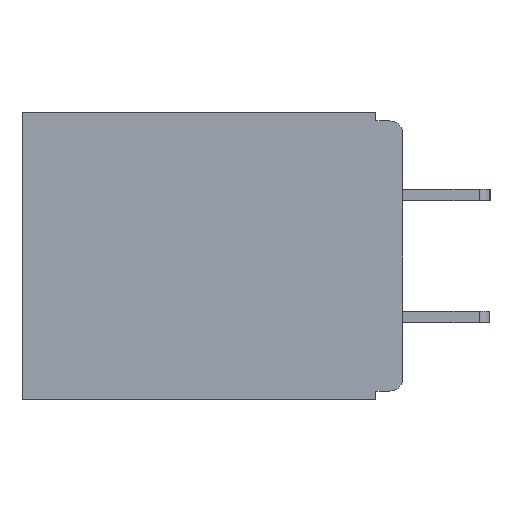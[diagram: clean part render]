
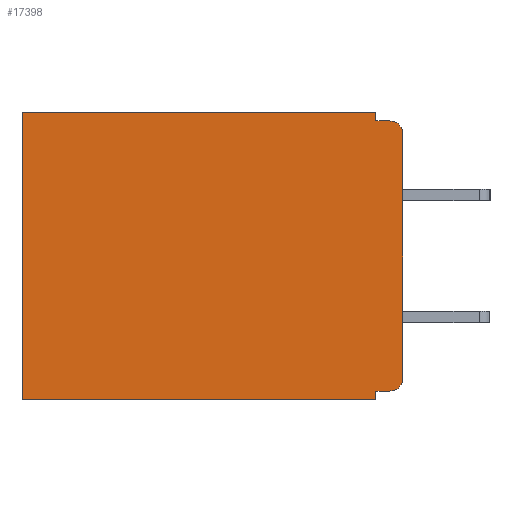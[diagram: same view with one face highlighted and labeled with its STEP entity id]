
A CAD part, left-side view. The second image highlights one B-rep face of the part: STEP entity #17398.
In plain terms, the highlighted planar face has unit normal (-1, 0, 0).
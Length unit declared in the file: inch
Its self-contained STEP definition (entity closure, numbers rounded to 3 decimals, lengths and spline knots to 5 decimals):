
#176 = CIRCLE ( 'NONE', #2695, 0.015 ) ;
#300 = ORIENTED_EDGE ( 'NONE', *, *, #22108, .F. ) ;
#583 = DIRECTION ( 'NONE',  ( 0., 0., -1. ) ) ;
#605 = DIRECTION ( 'NONE',  ( -1., 0., 0. ) ) ;
#666 = CARTESIAN_POINT ( 'NONE',  ( 0.3, 0.015, -0.305 ) ) ;
#902 = EDGE_CURVE ( 'NONE', #16992, #15504, #8045, .T. ) ;
#1127 = EDGE_CURVE ( 'NONE', #23476, #9948, #3181, .T. ) ;
#1251 = ORIENTED_EDGE ( 'NONE', *, *, #19569, .T. ) ;
#1346 = VECTOR ( 'NONE', #21164, 39.37008 ) ;
#1604 = CARTESIAN_POINT ( 'NONE',  ( 0.3, 0.015, -0.025 ) ) ;
#1906 = LINE ( 'NONE', #24030, #11576 ) ;
#1983 = VERTEX_POINT ( 'NONE', #21774 ) ;
#2018 = CARTESIAN_POINT ( 'NONE',  ( 0.3, 0., -0.32 ) ) ;
#2267 = VECTOR ( 'NONE', #6379, 39.37008 ) ;
#2303 = EDGE_LOOP ( 'NONE', ( #6532, #10044, #18871, #16533, #1251, #11111, #6105, #300, #2674, #8237 ) ) ;
#2674 = ORIENTED_EDGE ( 'NONE', *, *, #21019, .F. ) ;
#2695 = AXIS2_PLACEMENT_3D ( 'NONE', #666, #605, #583 ) ;
#3181 = LINE ( 'NONE', #22699, #8340 ) ;
#3318 = DIRECTION ( 'NONE',  ( 0., 0., -1. ) ) ;
#3605 = DIRECTION ( 'NONE',  ( 0., 0., -1. ) ) ;
#3680 = LINE ( 'NONE', #10888, #23286 ) ;
#3996 = DIRECTION ( 'NONE',  ( 0., 1., 0. ) ) ;
#4055 = CARTESIAN_POINT ( 'NONE',  ( 0.3, 0.437, 0. ) ) ;
#5127 = DIRECTION ( 'NONE',  ( 0., -1., 0. ) ) ;
#5719 = EDGE_CURVE ( 'NONE', #16009, #7254, #176, .T. ) ;
#5975 = DIRECTION ( 'NONE',  ( 0., 0., -1. ) ) ;
#6105 = ORIENTED_EDGE ( 'NONE', *, *, #20366, .F. ) ;
#6379 = DIRECTION ( 'NONE',  ( 0., 0., -1. ) ) ;
#6532 = ORIENTED_EDGE ( 'NONE', *, *, #16728, .F. ) ;
#6965 = VERTEX_POINT ( 'NONE', #15202 ) ;
#7078 = CARTESIAN_POINT ( 'NONE',  ( 0.3, 0., -0.33 ) ) ;
#7254 = VERTEX_POINT ( 'NONE', #21059 ) ;
#7880 = EDGE_CURVE ( 'NONE', #9948, #21154, #1906, .T. ) ;
#8045 = LINE ( 'NONE', #19472, #2267 ) ;
#8228 = CARTESIAN_POINT ( 'NONE',  ( 0.3, 0.015, -0.01 ) ) ;
#8237 = ORIENTED_EDGE ( 'NONE', *, *, #5719, .T. ) ;
#8340 = VECTOR ( 'NONE', #5975, 39.37008 ) ;
#9048 = DIRECTION ( 'NONE',  ( 1., 0., 0. ) ) ;
#9384 = CARTESIAN_POINT ( 'NONE',  ( 0.3, 0.031, -0.01 ) ) ;
#9879 = CARTESIAN_POINT ( 'NONE',  ( 0.3, 0., -0.33 ) ) ;
#9944 = LINE ( 'NONE', #11199, #19361 ) ;
#9948 = VERTEX_POINT ( 'NONE', #9384 ) ;
#10044 = ORIENTED_EDGE ( 'NONE', *, *, #14628, .T. ) ;
#10888 = CARTESIAN_POINT ( 'NONE',  ( 0.3, 0., -0.33 ) ) ;
#11111 = ORIENTED_EDGE ( 'NONE', *, *, #902, .T. ) ;
#11199 = CARTESIAN_POINT ( 'NONE',  ( 0.3, 0., 0. ) ) ;
#11576 = VECTOR ( 'NONE', #5127, 39.37008 ) ;
#11639 = LINE ( 'NONE', #9879, #1346 ) ;
#11655 = CARTESIAN_POINT ( 'NONE',  ( 0.3, 0.031, 0. ) ) ;
#14048 = CARTESIAN_POINT ( 'NONE',  ( 0.3, 0.437, -0.33 ) ) ;
#14628 = EDGE_CURVE ( 'NONE', #1983, #21154, #19047, .T. ) ;
#14981 = DIRECTION ( 'NONE',  ( -1., 0., 0. ) ) ;
#15202 = CARTESIAN_POINT ( 'NONE',  ( 0.3, 0.031, -0.32 ) ) ;
#15504 = VERTEX_POINT ( 'NONE', #14048 ) ;
#16009 = VERTEX_POINT ( 'NONE', #19448 ) ;
#16027 = CARTESIAN_POINT ( 'NONE',  ( 0.3, 0.031, -0.33 ) ) ;
#16530 = VECTOR ( 'NONE', #3318, 39.37008 ) ;
#16533 = ORIENTED_EDGE ( 'NONE', *, *, #1127, .F. ) ;
#16728 = EDGE_CURVE ( 'NONE', #1983, #7254, #3680, .T. ) ;
#16887 = LINE ( 'NONE', #2018, #17502 ) ;
#16992 = VERTEX_POINT ( 'NONE', #4055 ) ;
#17398 = ADVANCED_FACE ( 'NONE', ( #24116 ), #18427, .F. ) ;
#17502 = VECTOR ( 'NONE', #3996, 39.37008 ) ;
#18427 = PLANE ( 'NONE',  #22030 ) ;
#18459 = DIRECTION ( 'NONE',  ( 0., 0., -1. ) ) ;
#18553 = CARTESIAN_POINT ( 'NONE',  ( 0.3, 0.031, -0.33 ) ) ;
#18786 = DIRECTION ( 'NONE',  ( 0., 1., 0. ) ) ;
#18871 = ORIENTED_EDGE ( 'NONE', *, *, #7880, .F. ) ;
#19047 = CIRCLE ( 'NONE', #24143, 0.015 ) ;
#19361 = VECTOR ( 'NONE', #18786, 39.37008 ) ;
#19448 = CARTESIAN_POINT ( 'NONE',  ( 0.3, 0.015, -0.32 ) ) ;
#19472 = CARTESIAN_POINT ( 'NONE',  ( 0.3, 0.437, -0.33 ) ) ;
#19569 = EDGE_CURVE ( 'NONE', #23476, #16992, #9944, .T. ) ;
#20366 = EDGE_CURVE ( 'NONE', #24277, #15504, #11639, .T. ) ;
#21019 = EDGE_CURVE ( 'NONE', #16009, #6965, #16887, .T. ) ;
#21059 = CARTESIAN_POINT ( 'NONE',  ( 0.3, 0., -0.305 ) ) ;
#21154 = VERTEX_POINT ( 'NONE', #8228 ) ;
#21164 = DIRECTION ( 'NONE',  ( 0., 1., 0. ) ) ;
#21774 = CARTESIAN_POINT ( 'NONE',  ( 0.3, 0., -0.025 ) ) ;
#22030 = AXIS2_PLACEMENT_3D ( 'NONE', #7078, #9048, #22238 ) ;
#22108 = EDGE_CURVE ( 'NONE', #6965, #24277, #22175, .T. ) ;
#22175 = LINE ( 'NONE', #18553, #16530 ) ;
#22238 = DIRECTION ( 'NONE',  ( 0., 0., -1. ) ) ;
#22699 = CARTESIAN_POINT ( 'NONE',  ( 0.3, 0.031, 0. ) ) ;
#23286 = VECTOR ( 'NONE', #18459, 39.37008 ) ;
#23476 = VERTEX_POINT ( 'NONE', #11655 ) ;
#24030 = CARTESIAN_POINT ( 'NONE',  ( 0.3, 0., -0.01 ) ) ;
#24116 = FACE_OUTER_BOUND ( 'NONE', #2303, .T. ) ;
#24143 = AXIS2_PLACEMENT_3D ( 'NONE', #1604, #14981, #3605 ) ;
#24277 = VERTEX_POINT ( 'NONE', #16027 ) ;
